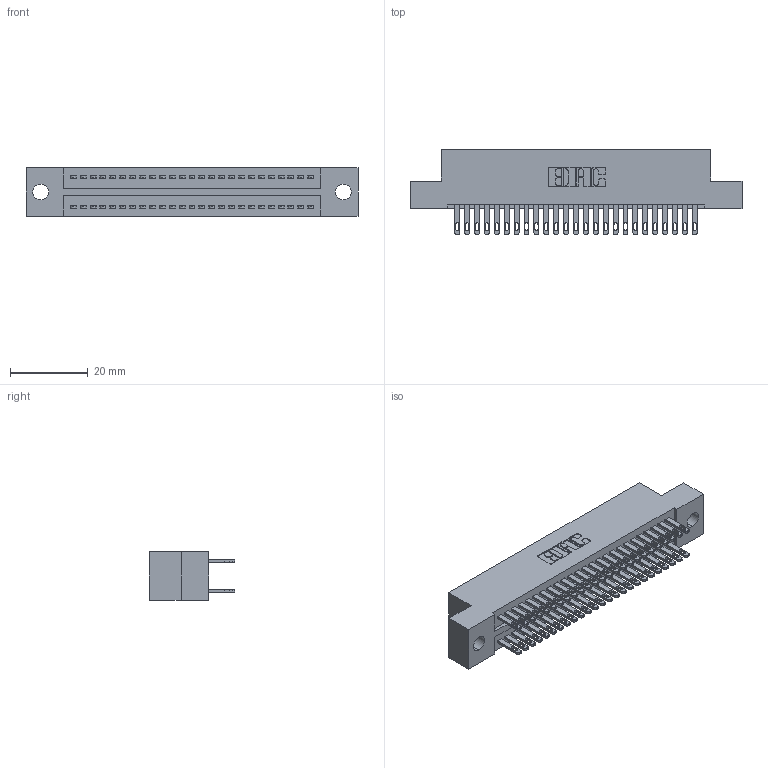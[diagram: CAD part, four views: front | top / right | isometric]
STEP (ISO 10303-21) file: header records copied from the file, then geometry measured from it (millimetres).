
FILE_DESCRIPTION (( 'STEP AP203' ), '1' );
FILE_NAME ('325-050-500-209.STEP', '2020-02-24T23:50:02', ( '' ), ( '' ), 'SwSTEP 2.0', 'SolidWorks 2016', '' );
FILE_SCHEMA (( 'CONFIG_CONTROL_DESIGN' ));
Length unit declared in the file: inch
Products named in the file (3): 325-292-001_325-293-100; 325-050-500-209; 325 Part_.160 TH
Assembly tree (51 placements, depth 2):
  325-050-500-209
    325 Part_.160 TH
    325-292-001_325-293-100  x50
Bounding box: 85.22 x 21.84 x 12.45 mm (x, y, z)
Volume: 10770.6 mm3; surface area: 13076.5 mm2
Topology: 51 solids, 51 shells, 2514 faces, 7661 edges, 5106 vertices
Faces by surface type: plane 1570, cylinder 944
Entity records: 18215 total; most frequent: CARTESIAN_POINT 3038, ORIENTED_EDGE 2974, DIRECTION 2627, EDGE_CURVE 1487, LINE 1355, VECTOR 1355, VERTEX_POINT 990, AXIS2_PLACEMENT_3D 636
